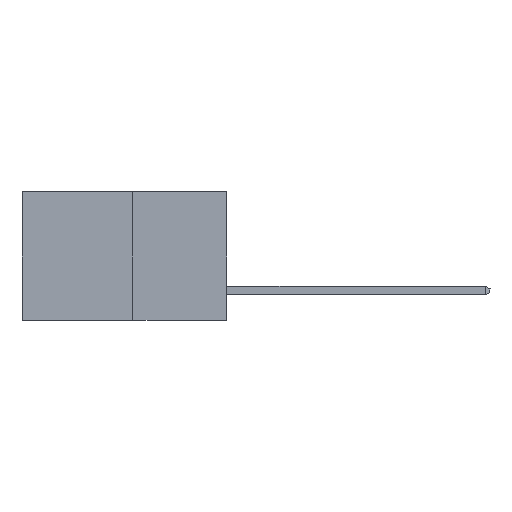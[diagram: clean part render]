
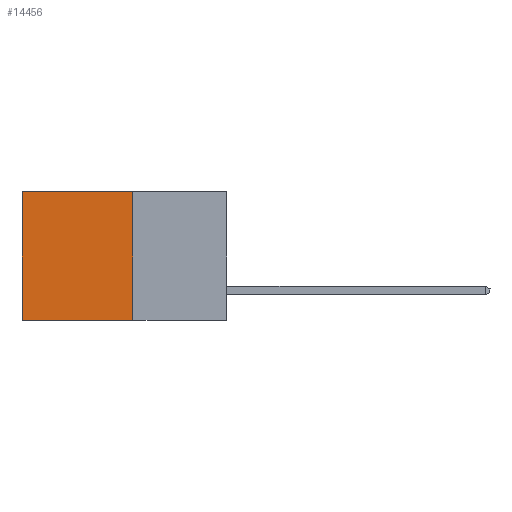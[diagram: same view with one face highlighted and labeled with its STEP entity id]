
A CAD part, left-side view. The second image highlights one B-rep face of the part: STEP entity #14456.
In plain terms, the highlighted planar face has unit normal (-1, 0, 0).
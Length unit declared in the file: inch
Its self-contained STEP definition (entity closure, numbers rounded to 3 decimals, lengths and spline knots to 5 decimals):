
#60 = VECTOR ( 'NONE', #1635, 39.37008 ) ;
#224 = VERTEX_POINT ( 'NONE', #5750 ) ;
#470 = DIRECTION ( 'NONE',  ( 0., 0., -1. ) ) ;
#1635 = DIRECTION ( 'NONE',  ( 0., 0., -1. ) ) ;
#1925 = CARTESIAN_POINT ( 'NONE',  ( 0.277, 0.27, -0.37 ) ) ;
#1966 = VECTOR ( 'NONE', #15066, 39.37008 ) ;
#2116 = CARTESIAN_POINT ( 'NONE',  ( 0.277, 0.27, 0. ) ) ;
#2300 = CARTESIAN_POINT ( 'NONE',  ( 0.277, 0.59, -0.37 ) ) ;
#3000 = EDGE_CURVE ( 'NONE', #7335, #224, #11399, .T. ) ;
#3369 = CARTESIAN_POINT ( 'NONE',  ( 0.277, 0.27, -0.37 ) ) ;
#3401 = EDGE_CURVE ( 'NONE', #11157, #11914, #3537, .T. ) ;
#3537 = LINE ( 'NONE', #2300, #60 ) ;
#4239 = CARTESIAN_POINT ( 'NONE',  ( 0.277, 0.59, -0.37 ) ) ;
#5056 = EDGE_LOOP ( 'NONE', ( #8479, #8494, #8593, #8605 ) ) ;
#5750 = CARTESIAN_POINT ( 'NONE',  ( 0.277, 0.27, -0.37 ) ) ;
#6422 = LINE ( 'NONE', #8711, #12786 ) ;
#7335 = VERTEX_POINT ( 'NONE', #2116 ) ;
#7363 = EDGE_CURVE ( 'NONE', #224, #11914, #11236, .T. ) ;
#8092 = DIRECTION ( 'NONE',  ( 1., 0., 0. ) ) ;
#8479 = ORIENTED_EDGE ( 'NONE', *, *, #3401, .T. ) ;
#8494 = ORIENTED_EDGE ( 'NONE', *, *, #7363, .F. ) ;
#8593 = ORIENTED_EDGE ( 'NONE', *, *, #3000, .F. ) ;
#8605 = ORIENTED_EDGE ( 'NONE', *, *, #14834, .T. ) ;
#8711 = CARTESIAN_POINT ( 'NONE',  ( 0.277, 0.27, 0. ) ) ;
#8757 = DIRECTION ( 'NONE',  ( 0., 1., 0. ) ) ;
#9083 = CARTESIAN_POINT ( 'NONE',  ( 0.277, 0.59, 0. ) ) ;
#10877 = VECTOR ( 'NONE', #8757, 39.37008 ) ;
#11009 = FACE_OUTER_BOUND ( 'NONE', #5056, .T. ) ;
#11157 = VERTEX_POINT ( 'NONE', #9083 ) ;
#11236 = LINE ( 'NONE', #3369, #10877 ) ;
#11399 = LINE ( 'NONE', #1925, #1966 ) ;
#11914 = VERTEX_POINT ( 'NONE', #4239 ) ;
#12353 = AXIS2_PLACEMENT_3D ( 'NONE', #12736, #8092, #470 ) ;
#12736 = CARTESIAN_POINT ( 'NONE',  ( 0.277, 0.27, -0.37 ) ) ;
#12786 = VECTOR ( 'NONE', #13261, 39.37008 ) ;
#13261 = DIRECTION ( 'NONE',  ( 0., 1., 0. ) ) ;
#14456 = ADVANCED_FACE ( 'NONE', ( #11009 ), #14733, .F. ) ;
#14733 = PLANE ( 'NONE',  #12353 ) ;
#14834 = EDGE_CURVE ( 'NONE', #7335, #11157, #6422, .T. ) ;
#15066 = DIRECTION ( 'NONE',  ( 0., 0., -1. ) ) ;
